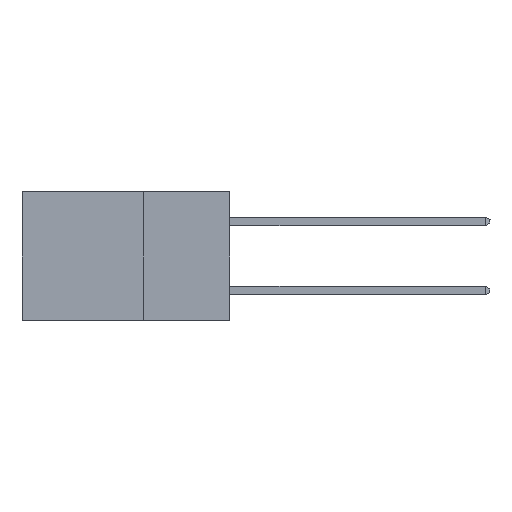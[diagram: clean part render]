
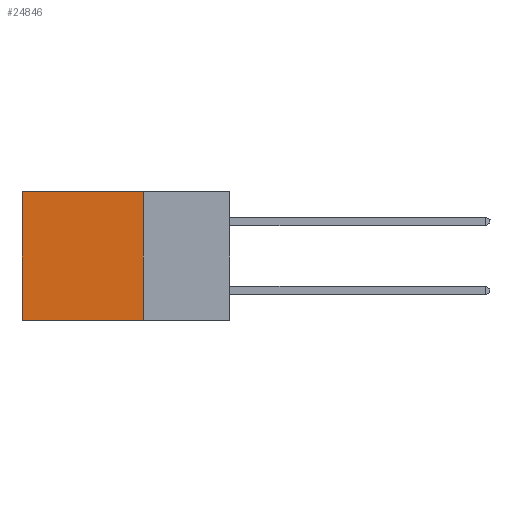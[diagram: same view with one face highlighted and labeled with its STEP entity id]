
A CAD part, left-side view. The second image highlights one B-rep face of the part: STEP entity #24846.
In plain terms, the highlighted planar face has unit normal (-1, 0, 0).
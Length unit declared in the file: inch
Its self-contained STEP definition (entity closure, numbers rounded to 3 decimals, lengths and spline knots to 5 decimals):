
#472 = DIRECTION ( 'NONE',  ( 0., 0., -1. ) ) ;
#1618 = ORIENTED_EDGE ( 'NONE', *, *, #3136, .F. ) ;
#1874 = CARTESIAN_POINT ( 'NONE',  ( 0.2615, 0.6, -0.37 ) ) ;
#1899 = CARTESIAN_POINT ( 'NONE',  ( 0.2615, 0.25, -0.37 ) ) ;
#2892 = VERTEX_POINT ( 'NONE', #21506 ) ;
#3009 = VECTOR ( 'NONE', #472, 39.37008 ) ;
#3136 = EDGE_CURVE ( 'NONE', #14373, #4930, #20664, .T. ) ;
#3582 = ORIENTED_EDGE ( 'NONE', *, *, #22850, .T. ) ;
#3981 = EDGE_CURVE ( 'NONE', #7052, #4930, #7359, .T. ) ;
#4930 = VERTEX_POINT ( 'NONE', #1874 ) ;
#5359 = CARTESIAN_POINT ( 'NONE',  ( 0.2615, 0.25, 0. ) ) ;
#6936 = ORIENTED_EDGE ( 'NONE', *, *, #3981, .T. ) ;
#7052 = VERTEX_POINT ( 'NONE', #16346 ) ;
#7359 = LINE ( 'NONE', #22239, #3009 ) ;
#8490 = ORIENTED_EDGE ( 'NONE', *, *, #26604, .F. ) ;
#11425 = VECTOR ( 'NONE', #20049, 39.37008 ) ;
#13609 = DIRECTION ( 'NONE',  ( 1., 0., 0. ) ) ;
#13757 = DIRECTION ( 'NONE',  ( 0., 0., -1. ) ) ;
#13998 = LINE ( 'NONE', #14150, #18592 ) ;
#14150 = CARTESIAN_POINT ( 'NONE',  ( 0.2615, 0.25, -0.37 ) ) ;
#14275 = EDGE_LOOP ( 'NONE', ( #6936, #1618, #8490, #3582 ) ) ;
#14373 = VERTEX_POINT ( 'NONE', #21081 ) ;
#16105 = DIRECTION ( 'NONE',  ( 0., 0., -1. ) ) ;
#16346 = CARTESIAN_POINT ( 'NONE',  ( 0.2615, 0.6, 0. ) ) ;
#17718 = VECTOR ( 'NONE', #18428, 39.37008 ) ;
#18428 = DIRECTION ( 'NONE',  ( 0., 1., 0. ) ) ;
#18592 = VECTOR ( 'NONE', #16105, 39.37008 ) ;
#20018 = PLANE ( 'NONE',  #26108 ) ;
#20049 = DIRECTION ( 'NONE',  ( 0., 1., 0. ) ) ;
#20664 = LINE ( 'NONE', #1899, #17718 ) ;
#21081 = CARTESIAN_POINT ( 'NONE',  ( 0.2615, 0.25, -0.37 ) ) ;
#21506 = CARTESIAN_POINT ( 'NONE',  ( 0.2615, 0.25, 0. ) ) ;
#22239 = CARTESIAN_POINT ( 'NONE',  ( 0.2615, 0.6, -0.37 ) ) ;
#22850 = EDGE_CURVE ( 'NONE', #2892, #7052, #26136, .T. ) ;
#24319 = FACE_OUTER_BOUND ( 'NONE', #14275, .T. ) ;
#24846 = ADVANCED_FACE ( 'NONE', ( #24319 ), #20018, .F. ) ;
#26108 = AXIS2_PLACEMENT_3D ( 'NONE', #26380, #13609, #13757 ) ;
#26136 = LINE ( 'NONE', #5359, #11425 ) ;
#26380 = CARTESIAN_POINT ( 'NONE',  ( 0.2615, 0.25, -0.37 ) ) ;
#26604 = EDGE_CURVE ( 'NONE', #2892, #14373, #13998, .T. ) ;
